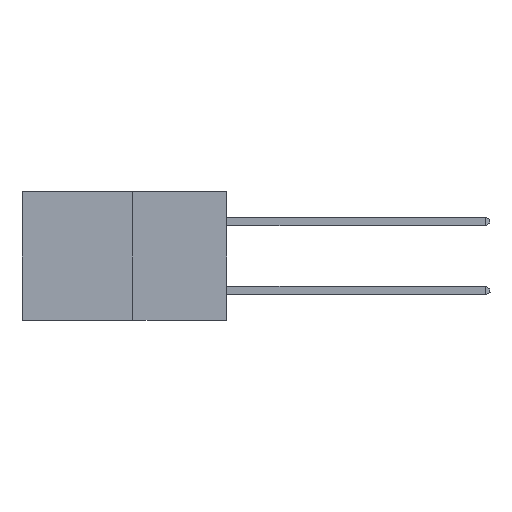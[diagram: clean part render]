
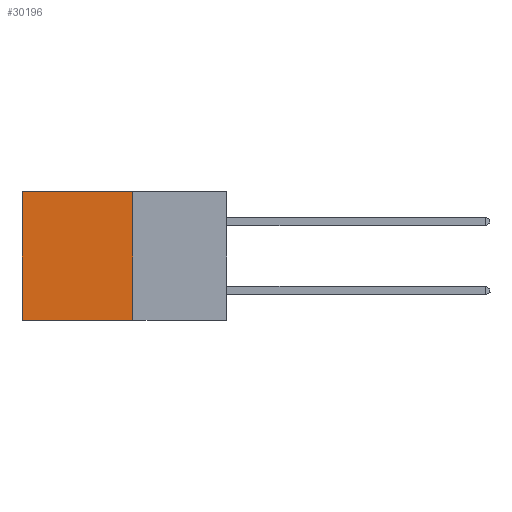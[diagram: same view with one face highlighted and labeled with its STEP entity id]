
A CAD part, left-side view. The second image highlights one B-rep face of the part: STEP entity #30196.
In plain terms, the highlighted planar face has unit normal (-1, 0, 0).
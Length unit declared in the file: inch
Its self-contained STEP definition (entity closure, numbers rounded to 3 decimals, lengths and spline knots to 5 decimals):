
#136 = VERTEX_POINT ( 'NONE', #10130 ) ;
#3632 = CARTESIAN_POINT ( 'NONE',  ( 0.277, 0.27, -0.37 ) ) ;
#4475 = DIRECTION ( 'NONE',  ( 0., 0., -1. ) ) ;
#4681 = LINE ( 'NONE', #15568, #12203 ) ;
#5038 = PLANE ( 'NONE',  #27240 ) ;
#5324 = VERTEX_POINT ( 'NONE', #20256 ) ;
#5898 = LINE ( 'NONE', #24698, #31768 ) ;
#7656 = EDGE_CURVE ( 'NONE', #14979, #136, #28910, .T. ) ;
#8851 = DIRECTION ( 'NONE',  ( 0., 1., 0. ) ) ;
#10130 = CARTESIAN_POINT ( 'NONE',  ( 0.277, 0.59, -0.37 ) ) ;
#11789 = ORIENTED_EDGE ( 'NONE', *, *, #19280, .F. ) ;
#11877 = ORIENTED_EDGE ( 'NONE', *, *, #26322, .T. ) ;
#12203 = VECTOR ( 'NONE', #12969, 39.37008 ) ;
#12465 = VECTOR ( 'NONE', #4475, 39.37008 ) ;
#12642 = CARTESIAN_POINT ( 'NONE',  ( 0.277, 0.27, -0.37 ) ) ;
#12969 = DIRECTION ( 'NONE',  ( 0., 1., 0. ) ) ;
#13148 = FACE_OUTER_BOUND ( 'NONE', #22337, .T. ) ;
#14979 = VERTEX_POINT ( 'NONE', #24498 ) ;
#15167 = DIRECTION ( 'NONE',  ( 0., 0., -1. ) ) ;
#15568 = CARTESIAN_POINT ( 'NONE',  ( 0.277, 0.27, 0. ) ) ;
#17754 = CARTESIAN_POINT ( 'NONE',  ( 0.277, 0.59, 0. ) ) ;
#19280 = EDGE_CURVE ( 'NONE', #5324, #14979, #19895, .T. ) ;
#19555 = CARTESIAN_POINT ( 'NONE',  ( 0.277, 0.27, -0.37 ) ) ;
#19895 = LINE ( 'NONE', #19555, #12465 ) ;
#20068 = VERTEX_POINT ( 'NONE', #17754 ) ;
#20256 = CARTESIAN_POINT ( 'NONE',  ( 0.277, 0.27, 0. ) ) ;
#22337 = EDGE_LOOP ( 'NONE', ( #27488, #27713, #11789, #11877 ) ) ;
#24498 = CARTESIAN_POINT ( 'NONE',  ( 0.277, 0.27, -0.37 ) ) ;
#24698 = CARTESIAN_POINT ( 'NONE',  ( 0.277, 0.59, -0.37 ) ) ;
#26017 = EDGE_CURVE ( 'NONE', #20068, #136, #5898, .T. ) ;
#26322 = EDGE_CURVE ( 'NONE', #5324, #20068, #4681, .T. ) ;
#27240 = AXIS2_PLACEMENT_3D ( 'NONE', #12642, #30150, #15167 ) ;
#27488 = ORIENTED_EDGE ( 'NONE', *, *, #26017, .T. ) ;
#27713 = ORIENTED_EDGE ( 'NONE', *, *, #7656, .F. ) ;
#28133 = VECTOR ( 'NONE', #8851, 39.37008 ) ;
#28910 = LINE ( 'NONE', #3632, #28133 ) ;
#29716 = DIRECTION ( 'NONE',  ( 0., 0., -1. ) ) ;
#30150 = DIRECTION ( 'NONE',  ( 1., 0., 0. ) ) ;
#30196 = ADVANCED_FACE ( 'NONE', ( #13148 ), #5038, .F. ) ;
#31768 = VECTOR ( 'NONE', #29716, 39.37008 ) ;
